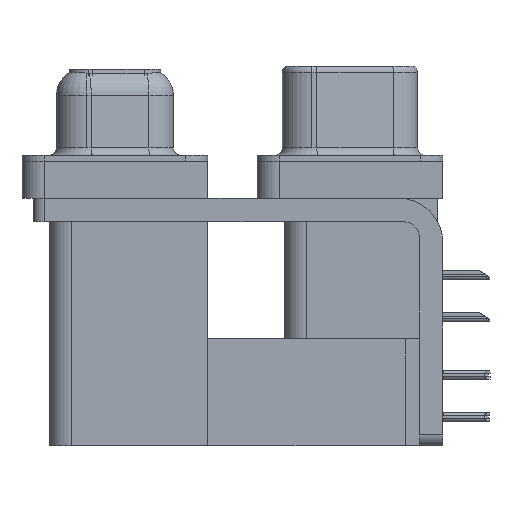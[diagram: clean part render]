
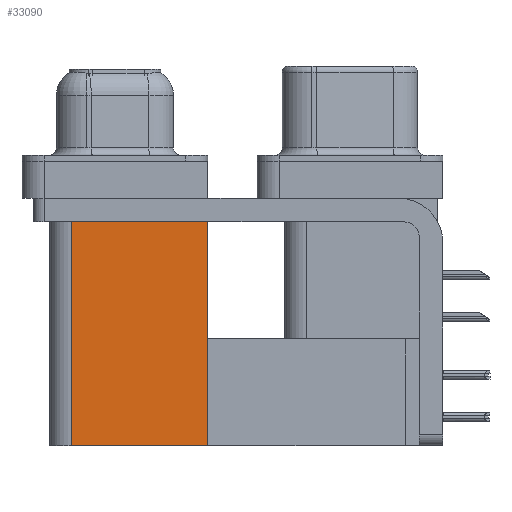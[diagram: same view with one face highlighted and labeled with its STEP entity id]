
A CAD part, left-side view. The second image highlights one B-rep face of the part: STEP entity #33090.
In plain terms, the highlighted planar face has unit normal (-1, 0, 0).
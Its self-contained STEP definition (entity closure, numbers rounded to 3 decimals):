
#24 = ORIENTED_EDGE ( 'NONE', *, *, #20233, .T. ) ;
#181 = VECTOR ( 'NONE', #3665, 1000. ) ;
#214 = AXIS2_PLACEMENT_3D ( 'NONE', #37267, #25031, #41520 ) ;
#2285 = VECTOR ( 'NONE', #22138, 1000. ) ;
#3665 = DIRECTION ( 'NONE',  ( 0., 1., 0. ) ) ;
#9457 = EDGE_CURVE ( 'NONE', #49368, #37925, #47649, .T. ) ;
#10987 = DIRECTION ( 'NONE',  ( 0., 0., 1. ) ) ;
#14466 = DIRECTION ( 'NONE',  ( 0., 1., 0. ) ) ;
#18447 = VECTOR ( 'NONE', #14466, 1000. ) ;
#20233 = EDGE_CURVE ( 'NONE', #49368, #40943, #52066, .T. ) ;
#21526 = CARTESIAN_POINT ( 'NONE',  ( 3.7, 18.8, -2.5 ) ) ;
#22138 = DIRECTION ( 'NONE',  ( 0., 0., 1. ) ) ;
#24766 = PLANE ( 'NONE',  #214 ) ;
#25031 = DIRECTION ( 'NONE',  ( 1., 0., 0. ) ) ;
#27776 = CARTESIAN_POINT ( 'NONE',  ( 3.7, 9.6, -2.5 ) ) ;
#28685 = EDGE_CURVE ( 'NONE', #37925, #48019, #35389, .T. ) ;
#30089 = CARTESIAN_POINT ( 'NONE',  ( 3.7, 9.6, -19.2 ) ) ;
#32112 = ORIENTED_EDGE ( 'NONE', *, *, #9457, .F. ) ;
#32670 = EDGE_CURVE ( 'NONE', #40943, #48019, #36533, .T. ) ;
#33090 = ADVANCED_FACE ( 'NONE', ( #33527 ), #24766, .F. ) ;
#33527 = FACE_OUTER_BOUND ( 'NONE', #49957, .T. ) ;
#34586 = CARTESIAN_POINT ( 'NONE',  ( 3.7, 9.6, -19.2 ) ) ;
#34735 = CARTESIAN_POINT ( 'NONE',  ( 3.7, 18.8, -19.2 ) ) ;
#35389 = LINE ( 'NONE', #43364, #45641 ) ;
#36533 = LINE ( 'NONE', #27776, #181 ) ;
#37267 = CARTESIAN_POINT ( 'NONE',  ( 3.7, 9.6, -19.2 ) ) ;
#37925 = VERTEX_POINT ( 'NONE', #34735 ) ;
#40121 = CARTESIAN_POINT ( 'NONE',  ( 3.7, 9.6, -2.5 ) ) ;
#40224 = ORIENTED_EDGE ( 'NONE', *, *, #28685, .F. ) ;
#40943 = VERTEX_POINT ( 'NONE', #40121 ) ;
#41520 = DIRECTION ( 'NONE',  ( 0., 0., -1. ) ) ;
#43364 = CARTESIAN_POINT ( 'NONE',  ( 3.7, 18.8, -19.2 ) ) ;
#43408 = CARTESIAN_POINT ( 'NONE',  ( 3.7, 9.6, -19.2 ) ) ;
#45641 = VECTOR ( 'NONE', #10987, 1000. ) ;
#47649 = LINE ( 'NONE', #43408, #18447 ) ;
#48019 = VERTEX_POINT ( 'NONE', #21526 ) ;
#48149 = ORIENTED_EDGE ( 'NONE', *, *, #32670, .T. ) ;
#49368 = VERTEX_POINT ( 'NONE', #34586 ) ;
#49957 = EDGE_LOOP ( 'NONE', ( #48149, #40224, #32112, #24 ) ) ;
#52066 = LINE ( 'NONE', #30089, #2285 ) ;
